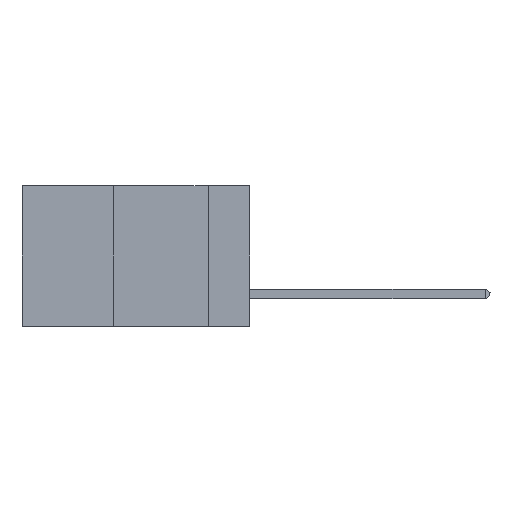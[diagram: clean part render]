
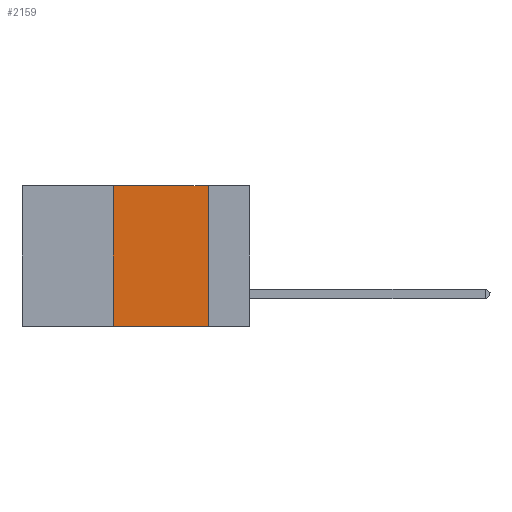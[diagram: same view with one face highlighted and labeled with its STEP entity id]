
A CAD part, left-side view. The second image highlights one B-rep face of the part: STEP entity #2159.
In plain terms, the highlighted planar face has unit normal (-1, 0, 0).
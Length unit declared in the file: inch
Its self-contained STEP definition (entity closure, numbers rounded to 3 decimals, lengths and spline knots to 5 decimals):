
#169 = ORIENTED_EDGE ( 'NONE', *, *, #6139, .F. ) ;
#254 = VECTOR ( 'NONE', #12390, 39.37008 ) ;
#541 = AXIS2_PLACEMENT_3D ( 'NONE', #14637, #12092, #10483 ) ;
#1635 = LINE ( 'NONE', #5473, #11963 ) ;
#1665 = VERTEX_POINT ( 'NONE', #2600 ) ;
#1950 = ORIENTED_EDGE ( 'NONE', *, *, #7917, .T. ) ;
#2034 = LINE ( 'NONE', #7248, #254 ) ;
#2159 = ADVANCED_FACE ( 'NONE', ( #13200 ), #10395, .F. ) ;
#2264 = VERTEX_POINT ( 'NONE', #12009 ) ;
#2600 = CARTESIAN_POINT ( 'NONE',  ( 0., 0.11, -0.37 ) ) ;
#5473 = CARTESIAN_POINT ( 'NONE',  ( 0., 0.11, 0. ) ) ;
#6139 = EDGE_CURVE ( 'NONE', #14349, #7794, #9513, .T. ) ;
#6152 = EDGE_CURVE ( 'NONE', #2264, #1665, #1635, .T. ) ;
#6575 = ORIENTED_EDGE ( 'NONE', *, *, #6152, .F. ) ;
#6847 = DIRECTION ( 'NONE',  ( 0., 0., -1. ) ) ;
#7233 = VECTOR ( 'NONE', #9899, 39.37008 ) ;
#7248 = CARTESIAN_POINT ( 'NONE',  ( 0., 0.6, -0.37 ) ) ;
#7794 = VERTEX_POINT ( 'NONE', #15011 ) ;
#7917 = EDGE_CURVE ( 'NONE', #14349, #1665, #2034, .T. ) ;
#8766 = ORIENTED_EDGE ( 'NONE', *, *, #10652, .F. ) ;
#8841 = EDGE_LOOP ( 'NONE', ( #6575, #8766, #169, #1950 ) ) ;
#9513 = LINE ( 'NONE', #11916, #15450 ) ;
#9899 = DIRECTION ( 'NONE',  ( 0., -1., 0. ) ) ;
#10395 = PLANE ( 'NONE',  #541 ) ;
#10483 = DIRECTION ( 'NONE',  ( 0., 0., -1. ) ) ;
#10652 = EDGE_CURVE ( 'NONE', #7794, #2264, #13812, .T. ) ;
#11916 = CARTESIAN_POINT ( 'NONE',  ( 0., 0.36, 0. ) ) ;
#11963 = VECTOR ( 'NONE', #6847, 39.37008 ) ;
#12009 = CARTESIAN_POINT ( 'NONE',  ( 0., 0.11, 0. ) ) ;
#12092 = DIRECTION ( 'NONE',  ( 1., 0., 0. ) ) ;
#12390 = DIRECTION ( 'NONE',  ( 0., -1., 0. ) ) ;
#12534 = CARTESIAN_POINT ( 'NONE',  ( 0., 0.6, 0. ) ) ;
#13200 = FACE_OUTER_BOUND ( 'NONE', #8841, .T. ) ;
#13812 = LINE ( 'NONE', #12534, #7233 ) ;
#14349 = VERTEX_POINT ( 'NONE', #14491 ) ;
#14491 = CARTESIAN_POINT ( 'NONE',  ( 0., 0.36, -0.37 ) ) ;
#14546 = DIRECTION ( 'NONE',  ( 0., 0., 1. ) ) ;
#14637 = CARTESIAN_POINT ( 'NONE',  ( 0., 0.6, 0. ) ) ;
#15011 = CARTESIAN_POINT ( 'NONE',  ( 0., 0.36, 0. ) ) ;
#15450 = VECTOR ( 'NONE', #14546, 39.37008 ) ;
